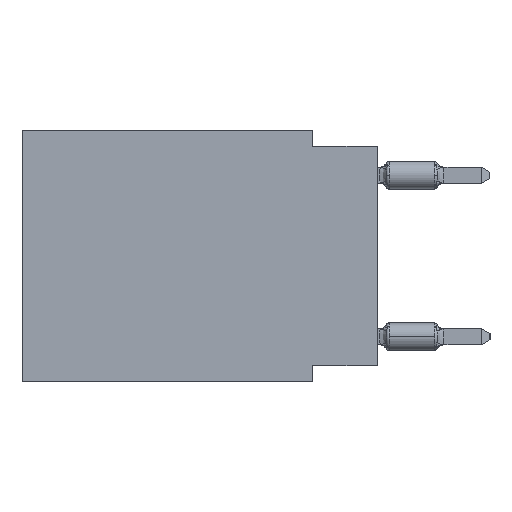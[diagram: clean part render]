
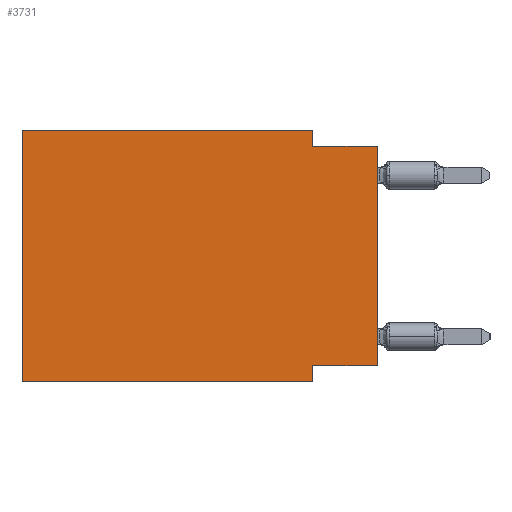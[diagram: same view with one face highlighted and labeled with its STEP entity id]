
A CAD part, left-side view. The second image highlights one B-rep face of the part: STEP entity #3731.
In plain terms, the highlighted planar face has unit normal (-1, 0, 0).
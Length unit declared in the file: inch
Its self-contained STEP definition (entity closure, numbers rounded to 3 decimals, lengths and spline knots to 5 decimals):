
#269 = FACE_OUTER_BOUND ( 'NONE', #20991, .T. ) ;
#299 = EDGE_CURVE ( 'NONE', #10442, #18524, #13113, .T. ) ;
#607 = VECTOR ( 'NONE', #5832, 39.37008 ) ;
#879 = LINE ( 'NONE', #4694, #11953 ) ;
#894 = CARTESIAN_POINT ( 'NONE',  ( 0., 0., -0.365 ) ) ;
#945 = CARTESIAN_POINT ( 'NONE',  ( 0., 0.55, -0.39 ) ) ;
#1094 = DIRECTION ( 'NONE',  ( 0., 0., -1. ) ) ;
#1585 = ORIENTED_EDGE ( 'NONE', *, *, #299, .F. ) ;
#1659 = VECTOR ( 'NONE', #12556, 39.37008 ) ;
#1694 = CARTESIAN_POINT ( 'NONE',  ( 0., 0.1, -0.39 ) ) ;
#1884 = VERTEX_POINT ( 'NONE', #10811 ) ;
#2020 = ORIENTED_EDGE ( 'NONE', *, *, #19514, .F. ) ;
#2098 = CARTESIAN_POINT ( 'NONE',  ( 0., 0.55, 0. ) ) ;
#2555 = CARTESIAN_POINT ( 'NONE',  ( 0., 0.55, -0.39 ) ) ;
#2887 = DIRECTION ( 'NONE',  ( 0., -1., 0. ) ) ;
#2924 = CARTESIAN_POINT ( 'NONE',  ( 0., 0., 0. ) ) ;
#3075 = ORIENTED_EDGE ( 'NONE', *, *, #13036, .F. ) ;
#3158 = DIRECTION ( 'NONE',  ( 0., 0., -1. ) ) ;
#3380 = CARTESIAN_POINT ( 'NONE',  ( 0., 0.1, -0.39 ) ) ;
#3420 = DIRECTION ( 'NONE',  ( 0., 0., 1. ) ) ;
#3660 = ORIENTED_EDGE ( 'NONE', *, *, #15555, .T. ) ;
#3731 = ADVANCED_FACE ( 'NONE', ( #269 ), #15295, .F. ) ;
#3971 = EDGE_CURVE ( 'NONE', #17404, #10442, #17346, .T. ) ;
#4494 = VECTOR ( 'NONE', #12363, 39.37008 ) ;
#4694 = CARTESIAN_POINT ( 'NONE',  ( 0., 0.1, 0. ) ) ;
#5016 = VECTOR ( 'NONE', #20390, 39.37008 ) ;
#5338 = VERTEX_POINT ( 'NONE', #2555 ) ;
#5461 = LINE ( 'NONE', #18233, #17798 ) ;
#5766 = CARTESIAN_POINT ( 'NONE',  ( 0., 0.55, 0. ) ) ;
#5807 = CARTESIAN_POINT ( 'NONE',  ( 0., 0.55, 0. ) ) ;
#5832 = DIRECTION ( 'NONE',  ( 0., -1., 0. ) ) ;
#6014 = VERTEX_POINT ( 'NONE', #8885 ) ;
#6617 = EDGE_CURVE ( 'NONE', #1884, #17162, #17703, .T. ) ;
#7368 = LINE ( 'NONE', #5766, #4494 ) ;
#8885 = CARTESIAN_POINT ( 'NONE',  ( 0., 0.1, 0. ) ) ;
#9294 = ORIENTED_EDGE ( 'NONE', *, *, #16009, .T. ) ;
#10329 = EDGE_CURVE ( 'NONE', #5338, #16337, #5461, .T. ) ;
#10442 = VERTEX_POINT ( 'NONE', #20375 ) ;
#10811 = CARTESIAN_POINT ( 'NONE',  ( 0., 0.1, -0.025 ) ) ;
#11210 = AXIS2_PLACEMENT_3D ( 'NONE', #2098, #18444, #20295 ) ;
#11953 = VECTOR ( 'NONE', #1094, 39.37008 ) ;
#12091 = CARTESIAN_POINT ( 'NONE',  ( 0., 0., -0.365 ) ) ;
#12363 = DIRECTION ( 'NONE',  ( 0., -1., 0. ) ) ;
#12556 = DIRECTION ( 'NONE',  ( 0., 0., 1. ) ) ;
#13036 = EDGE_CURVE ( 'NONE', #6014, #1884, #879, .T. ) ;
#13113 = LINE ( 'NONE', #3380, #16473 ) ;
#13666 = VECTOR ( 'NONE', #2887, 39.37008 ) ;
#15295 = PLANE ( 'NONE',  #11210 ) ;
#15555 = EDGE_CURVE ( 'NONE', #17404, #17162, #19382, .T. ) ;
#16009 = EDGE_CURVE ( 'NONE', #5338, #18524, #20645, .T. ) ;
#16087 = ORIENTED_EDGE ( 'NONE', *, *, #3971, .F. ) ;
#16337 = VERTEX_POINT ( 'NONE', #5807 ) ;
#16473 = VECTOR ( 'NONE', #3158, 39.37008 ) ;
#17162 = VERTEX_POINT ( 'NONE', #19134 ) ;
#17346 = LINE ( 'NONE', #894, #5016 ) ;
#17380 = CARTESIAN_POINT ( 'NONE',  ( 0., 0., -0.025 ) ) ;
#17404 = VERTEX_POINT ( 'NONE', #12091 ) ;
#17703 = LINE ( 'NONE', #17380, #13666 ) ;
#17798 = VECTOR ( 'NONE', #3420, 39.37008 ) ;
#17869 = ORIENTED_EDGE ( 'NONE', *, *, #10329, .F. ) ;
#18233 = CARTESIAN_POINT ( 'NONE',  ( 0., 0.55, 0. ) ) ;
#18444 = DIRECTION ( 'NONE',  ( 1., 0., 0. ) ) ;
#18524 = VERTEX_POINT ( 'NONE', #1694 ) ;
#19134 = CARTESIAN_POINT ( 'NONE',  ( 0., 0., -0.025 ) ) ;
#19382 = LINE ( 'NONE', #2924, #1659 ) ;
#19514 = EDGE_CURVE ( 'NONE', #16337, #6014, #7368, .T. ) ;
#19629 = ORIENTED_EDGE ( 'NONE', *, *, #6617, .F. ) ;
#20295 = DIRECTION ( 'NONE',  ( 0., 0., -1. ) ) ;
#20375 = CARTESIAN_POINT ( 'NONE',  ( 0., 0.1, -0.365 ) ) ;
#20390 = DIRECTION ( 'NONE',  ( 0., 1., 0. ) ) ;
#20645 = LINE ( 'NONE', #945, #607 ) ;
#20991 = EDGE_LOOP ( 'NONE', ( #3660, #19629, #3075, #2020, #17869, #9294, #1585, #16087 ) ) ;
